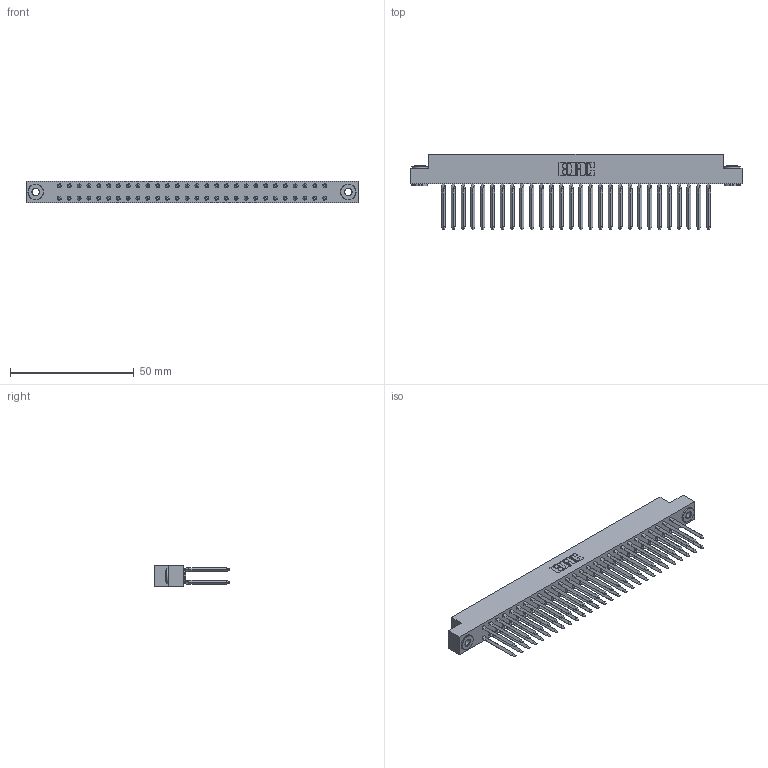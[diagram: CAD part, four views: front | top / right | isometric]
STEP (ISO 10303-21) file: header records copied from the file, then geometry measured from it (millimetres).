
FILE_DESCRIPTION (( 'STEP AP203' ), '1' );
FILE_NAME ('338-056-541-203.STEP', '2020-03-24T18:54:54', ( '' ), ( '' ), 'SwSTEP 2.0', 'SolidWorks 2016', '' );
FILE_SCHEMA (( 'CONFIG_CONTROL_DESIGN' ));
Length unit declared in the file: inch
Products named in the file (4): 338-290-001_541; 345-250-002_345-250-002-102; 338-056-541-203; 338-210-001_338-210-028-004
Assembly tree (59 placements, depth 2):
  338-056-541-203
    338-210-001_338-210-028-004
    338-290-001_541  x56
    345-250-002_345-250-002-102  x2
Bounding box: 133.96 x 30.56 x 8.71 mm (x, y, z)
Volume: 10357.2 mm3; surface area: 19763 mm2
Topology: 59 solids, 59 shells, 3898 faces, 10443 edges, 6622 vertices
Faces by surface type: plane 2706, cylinder 960, bspline 224, cone 8
Entity records: 57073 total; most frequent: CARTESIAN_POINT 11261, ORIENTED_EDGE 9480, DIRECTION 8925, EDGE_CURVE 4740, VECTOR 3537, LINE 3537, VERTEX_POINT 3078, AXIS2_PLACEMENT_3D 2694
